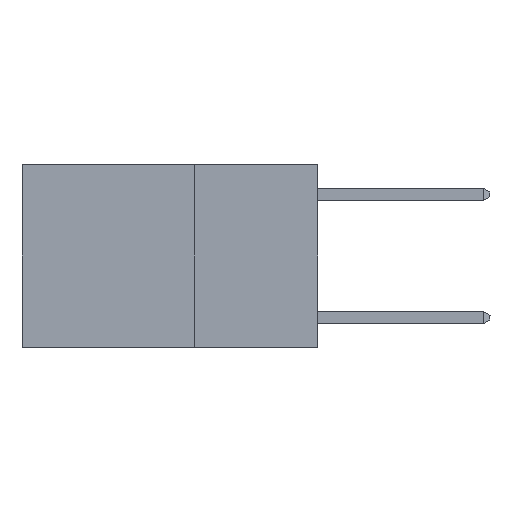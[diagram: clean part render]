
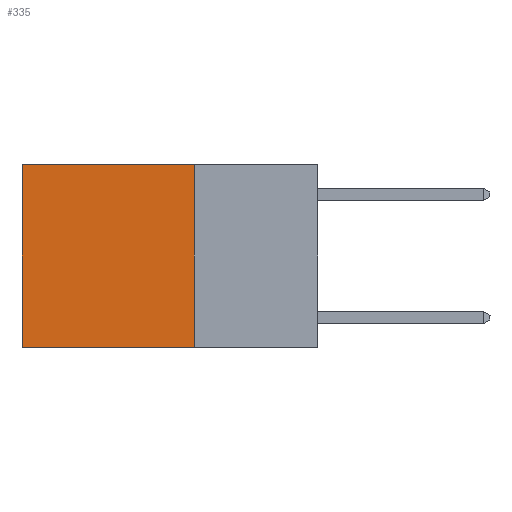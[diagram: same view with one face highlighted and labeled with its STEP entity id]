
A CAD part, left-side view. The second image highlights one B-rep face of the part: STEP entity #335.
In plain terms, the highlighted planar face has unit normal (-1, 0, 0).
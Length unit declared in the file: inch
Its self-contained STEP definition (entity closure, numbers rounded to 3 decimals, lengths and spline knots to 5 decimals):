
#335 = ADVANCED_FACE ( 'NONE', ( #23090 ), #24275, .F. ) ;
#598 = EDGE_CURVE ( 'NONE', #19486, #13732, #6371, .T. ) ;
#1028 = EDGE_CURVE ( 'NONE', #14062, #19486, #24585, .T. ) ;
#2727 = ORIENTED_EDGE ( 'NONE', *, *, #12206, .T. ) ;
#4012 = EDGE_LOOP ( 'NONE', ( #2727, #16929, #5486, #21617 ) ) ;
#5486 = ORIENTED_EDGE ( 'NONE', *, *, #1028, .F. ) ;
#5866 = VECTOR ( 'NONE', #23274, 39.37008 ) ;
#6371 = LINE ( 'NONE', #21098, #16785 ) ;
#6534 = LINE ( 'NONE', #17157, #5866 ) ;
#6720 = EDGE_CURVE ( 'NONE', #14062, #17571, #6534, .T. ) ;
#7423 = DIRECTION ( 'NONE',  ( 0., 0., -1. ) ) ;
#7927 = CARTESIAN_POINT ( 'NONE',  ( 0.2625, 0.25, 0. ) ) ;
#9188 = VECTOR ( 'NONE', #7423, 39.37008 ) ;
#9700 = CARTESIAN_POINT ( 'NONE',  ( 0.2625, 0.6, 0. ) ) ;
#9822 = LINE ( 'NONE', #23714, #9188 ) ;
#12206 = EDGE_CURVE ( 'NONE', #17571, #13732, #9822, .T. ) ;
#12335 = CARTESIAN_POINT ( 'NONE',  ( 0.2625, 0.25, 0. ) ) ;
#13732 = VERTEX_POINT ( 'NONE', #22007 ) ;
#14062 = VERTEX_POINT ( 'NONE', #17310 ) ;
#14178 = DIRECTION ( 'NONE',  ( 0., 0., -1. ) ) ;
#15395 = DIRECTION ( 'NONE',  ( 0., 1., 0. ) ) ;
#16785 = VECTOR ( 'NONE', #15395, 39.37008 ) ;
#16929 = ORIENTED_EDGE ( 'NONE', *, *, #598, .F. ) ;
#17157 = CARTESIAN_POINT ( 'NONE',  ( 0.2625, 0.25, 0. ) ) ;
#17310 = CARTESIAN_POINT ( 'NONE',  ( 0.2625, 0.25, 0. ) ) ;
#17571 = VERTEX_POINT ( 'NONE', #9700 ) ;
#19327 = VECTOR ( 'NONE', #26438, 39.37008 ) ;
#19486 = VERTEX_POINT ( 'NONE', #20108 ) ;
#20108 = CARTESIAN_POINT ( 'NONE',  ( 0.2625, 0.25, -0.37 ) ) ;
#21098 = CARTESIAN_POINT ( 'NONE',  ( 0.2625, 0.25, -0.37 ) ) ;
#21617 = ORIENTED_EDGE ( 'NONE', *, *, #6720, .T. ) ;
#22007 = CARTESIAN_POINT ( 'NONE',  ( 0.2625, 0.6, -0.37 ) ) ;
#22174 = AXIS2_PLACEMENT_3D ( 'NONE', #7927, #26230, #14178 ) ;
#23090 = FACE_OUTER_BOUND ( 'NONE', #4012, .T. ) ;
#23274 = DIRECTION ( 'NONE',  ( 0., 1., 0. ) ) ;
#23714 = CARTESIAN_POINT ( 'NONE',  ( 0.2625, 0.6, 0. ) ) ;
#24275 = PLANE ( 'NONE',  #22174 ) ;
#24585 = LINE ( 'NONE', #12335, #19327 ) ;
#26230 = DIRECTION ( 'NONE',  ( 1., 0., 0. ) ) ;
#26438 = DIRECTION ( 'NONE',  ( 0., 0., -1. ) ) ;
